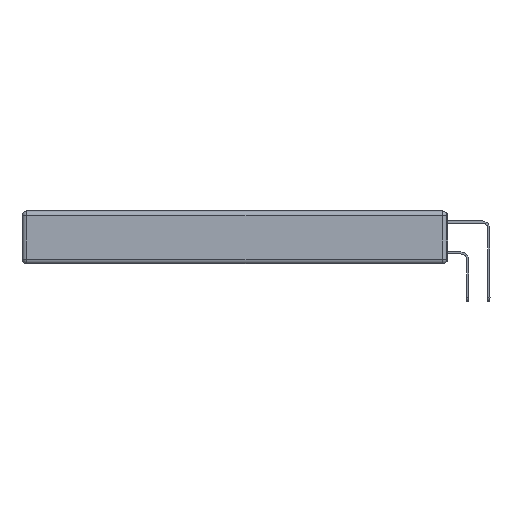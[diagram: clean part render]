
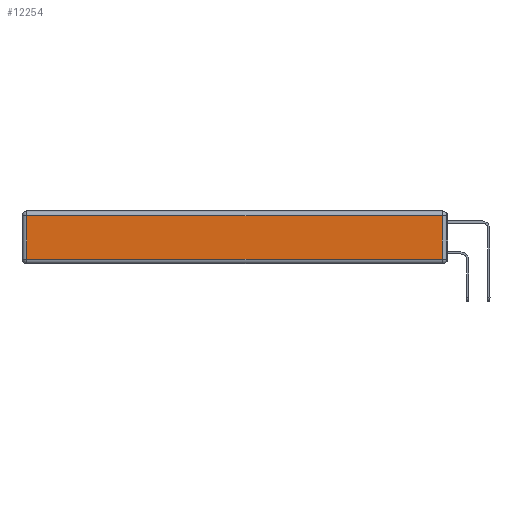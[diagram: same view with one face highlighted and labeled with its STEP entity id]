
A CAD part, left-side view. The second image highlights one B-rep face of the part: STEP entity #12254.
In plain terms, the highlighted planar face has unit normal (-1, 0, 0).
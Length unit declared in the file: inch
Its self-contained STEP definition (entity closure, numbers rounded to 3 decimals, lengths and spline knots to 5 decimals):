
#1006 = PLANE ( 'NONE',  #14979 ) ;
#1871 = VERTEX_POINT ( 'NONE', #9219 ) ;
#4946 = DIRECTION ( 'NONE',  ( 0., -1., 0. ) ) ;
#5372 = EDGE_CURVE ( 'NONE', #20054, #26756, #8725, .T. ) ;
#7117 = LINE ( 'NONE', #15947, #27739 ) ;
#8167 = CARTESIAN_POINT ( 'NONE',  ( 0., 2.72, -0.343 ) ) ;
#8340 = VECTOR ( 'NONE', #19280, 39.37008 ) ;
#8725 = LINE ( 'NONE', #26313, #23591 ) ;
#9219 = CARTESIAN_POINT ( 'NONE',  ( 0., 2.72, -0.313 ) ) ;
#9766 = EDGE_CURVE ( 'NONE', #23315, #20054, #14954, .T. ) ;
#12254 = ADVANCED_FACE ( 'NONE', ( #20379 ), #1006, .T. ) ;
#13426 = CARTESIAN_POINT ( 'NONE',  ( 0., 0.03, -0.03 ) ) ;
#13687 = ORIENTED_EDGE ( 'NONE', *, *, #5372, .T. ) ;
#14349 = EDGE_LOOP ( 'NONE', ( #20625, #27519, #13687, #14687 ) ) ;
#14687 = ORIENTED_EDGE ( 'NONE', *, *, #25041, .T. ) ;
#14954 = LINE ( 'NONE', #22005, #22248 ) ;
#14979 = AXIS2_PLACEMENT_3D ( 'NONE', #18373, #16481, #25132 ) ;
#15348 = DIRECTION ( 'NONE',  ( 0., 1., 0. ) ) ;
#15947 = CARTESIAN_POINT ( 'NONE',  ( 0., 0., -0.313 ) ) ;
#16481 = DIRECTION ( 'NONE',  ( -1., 0., 0. ) ) ;
#17557 = CARTESIAN_POINT ( 'NONE',  ( 0., 0.03, -0.313 ) ) ;
#18373 = CARTESIAN_POINT ( 'NONE',  ( 0., 0., -0.343 ) ) ;
#19280 = DIRECTION ( 'NONE',  ( 0., 0., -1. ) ) ;
#20054 = VERTEX_POINT ( 'NONE', #13426 ) ;
#20379 = FACE_OUTER_BOUND ( 'NONE', #14349, .T. ) ;
#20625 = ORIENTED_EDGE ( 'NONE', *, *, #26703, .T. ) ;
#20840 = LINE ( 'NONE', #8167, #8340 ) ;
#21585 = DIRECTION ( 'NONE',  ( 0., 0., 1. ) ) ;
#22005 = CARTESIAN_POINT ( 'NONE',  ( 0., 0.03, -0.343 ) ) ;
#22248 = VECTOR ( 'NONE', #21585, 39.37008 ) ;
#23315 = VERTEX_POINT ( 'NONE', #17557 ) ;
#23591 = VECTOR ( 'NONE', #15348, 39.37008 ) ;
#25041 = EDGE_CURVE ( 'NONE', #26756, #1871, #20840, .T. ) ;
#25132 = DIRECTION ( 'NONE',  ( 0., 0., 1. ) ) ;
#25724 = CARTESIAN_POINT ( 'NONE',  ( 0., 2.72, -0.03 ) ) ;
#26313 = CARTESIAN_POINT ( 'NONE',  ( 0., 2.75, -0.03 ) ) ;
#26703 = EDGE_CURVE ( 'NONE', #1871, #23315, #7117, .T. ) ;
#26756 = VERTEX_POINT ( 'NONE', #25724 ) ;
#27519 = ORIENTED_EDGE ( 'NONE', *, *, #9766, .T. ) ;
#27739 = VECTOR ( 'NONE', #4946, 39.37008 ) ;
